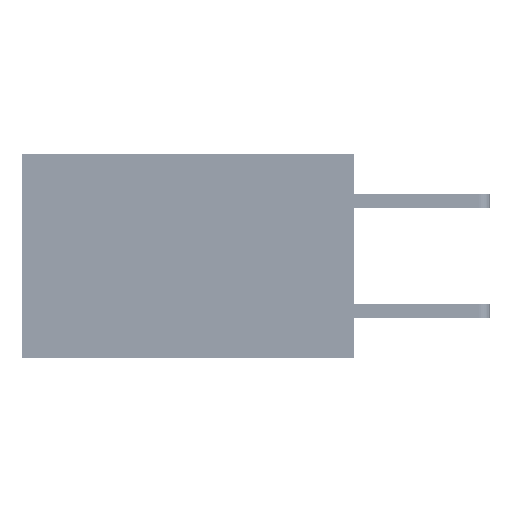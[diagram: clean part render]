
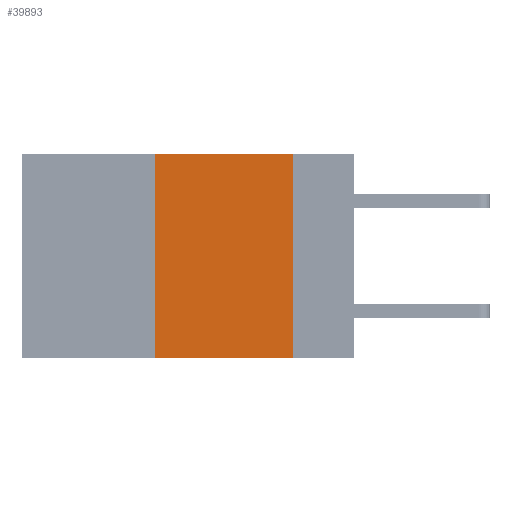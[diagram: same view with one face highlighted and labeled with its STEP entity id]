
A CAD part, left-side view. The second image highlights one B-rep face of the part: STEP entity #39893.
In plain terms, the highlighted planar face has unit normal (-1, 0, 0).
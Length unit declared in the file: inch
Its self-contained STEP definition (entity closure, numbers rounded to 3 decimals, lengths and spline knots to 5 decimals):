
#517 = DIRECTION ( 'NONE',  ( 0., 0., 1. ) ) ;
#1863 = EDGE_CURVE ( 'NONE', #9876, #7644, #36000, .T. ) ;
#2541 = DIRECTION ( 'NONE',  ( 0., -1., 0. ) ) ;
#3565 = ORIENTED_EDGE ( 'NONE', *, *, #1863, .T. ) ;
#4281 = CARTESIAN_POINT ( 'NONE',  ( 0., 0.11, 0. ) ) ;
#5431 = PLANE ( 'NONE',  #39743 ) ;
#5845 = VECTOR ( 'NONE', #517, 39.37008 ) ;
#6195 = DIRECTION ( 'NONE',  ( 1., 0., 0. ) ) ;
#7644 = VERTEX_POINT ( 'NONE', #7750 ) ;
#7750 = CARTESIAN_POINT ( 'NONE',  ( 0., 0.11, -0.37 ) ) ;
#8200 = LINE ( 'NONE', #23778, #5845 ) ;
#8675 = VECTOR ( 'NONE', #48254, 39.37008 ) ;
#8926 = CARTESIAN_POINT ( 'NONE',  ( 0., 0.6, -0.37 ) ) ;
#9876 = VERTEX_POINT ( 'NONE', #25266 ) ;
#10743 = ORIENTED_EDGE ( 'NONE', *, *, #39356, .F. ) ;
#13348 = CARTESIAN_POINT ( 'NONE',  ( 0., 0.6, 0. ) ) ;
#15808 = VERTEX_POINT ( 'NONE', #4281 ) ;
#15980 = LINE ( 'NONE', #27736, #34814 ) ;
#17430 = DIRECTION ( 'NONE',  ( 0., 0., -1. ) ) ;
#23743 = VERTEX_POINT ( 'NONE', #34230 ) ;
#23778 = CARTESIAN_POINT ( 'NONE',  ( 0., 0.36, 0. ) ) ;
#24009 = LINE ( 'NONE', #39597, #24955 ) ;
#24955 = VECTOR ( 'NONE', #2541, 39.37008 ) ;
#25266 = CARTESIAN_POINT ( 'NONE',  ( 0., 0.36, -0.37 ) ) ;
#27736 = CARTESIAN_POINT ( 'NONE',  ( 0., 0.11, 0. ) ) ;
#27956 = ORIENTED_EDGE ( 'NONE', *, *, #44306, .F. ) ;
#28753 = EDGE_CURVE ( 'NONE', #23743, #15808, #24009, .T. ) ;
#34230 = CARTESIAN_POINT ( 'NONE',  ( 0., 0.36, 0. ) ) ;
#34814 = VECTOR ( 'NONE', #44324, 39.37008 ) ;
#36000 = LINE ( 'NONE', #8926, #8675 ) ;
#36586 = FACE_OUTER_BOUND ( 'NONE', #40272, .T. ) ;
#39356 = EDGE_CURVE ( 'NONE', #15808, #7644, #15980, .T. ) ;
#39597 = CARTESIAN_POINT ( 'NONE',  ( 0., 0.6, 0. ) ) ;
#39743 = AXIS2_PLACEMENT_3D ( 'NONE', #13348, #6195, #17430 ) ;
#39893 = ADVANCED_FACE ( 'NONE', ( #36586 ), #5431, .F. ) ;
#40272 = EDGE_LOOP ( 'NONE', ( #10743, #40575, #27956, #3565 ) ) ;
#40575 = ORIENTED_EDGE ( 'NONE', *, *, #28753, .F. ) ;
#44306 = EDGE_CURVE ( 'NONE', #9876, #23743, #8200, .T. ) ;
#44324 = DIRECTION ( 'NONE',  ( 0., 0., -1. ) ) ;
#48254 = DIRECTION ( 'NONE',  ( 0., -1., 0. ) ) ;
